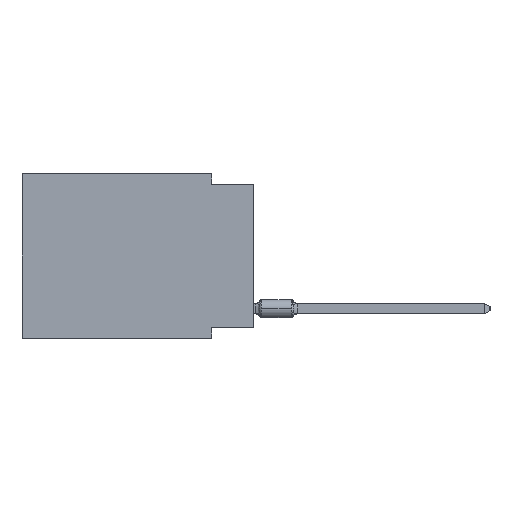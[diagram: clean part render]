
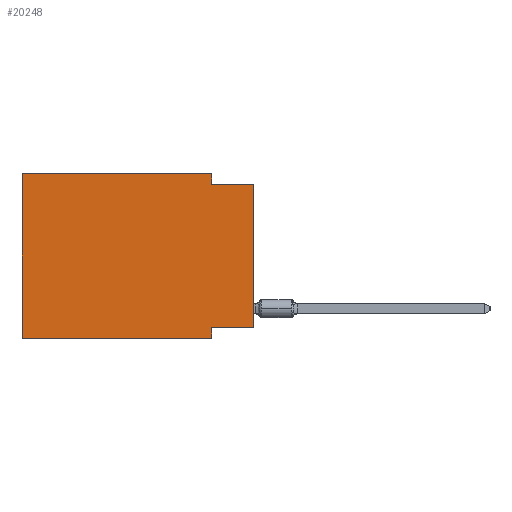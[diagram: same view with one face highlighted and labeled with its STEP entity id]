
A CAD part, left-side view. The second image highlights one B-rep face of the part: STEP entity #20248.
In plain terms, the highlighted planar face has unit normal (-1, 0, 0).
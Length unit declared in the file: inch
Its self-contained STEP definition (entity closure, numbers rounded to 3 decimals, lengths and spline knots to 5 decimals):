
#66 = LINE ( 'NONE', #49662, #8946 ) ;
#1656 = LINE ( 'NONE', #46971, #32949 ) ;
#2371 = DIRECTION ( 'NONE',  ( 0., 0., -1. ) ) ;
#3465 = DIRECTION ( 'NONE',  ( 0., 1., 0. ) ) ;
#4087 = ORIENTED_EDGE ( 'NONE', *, *, #4797, .F. ) ;
#4797 = EDGE_CURVE ( 'NONE', #6938, #42420, #9261, .T. ) ;
#4893 = FACE_OUTER_BOUND ( 'NONE', #39139, .T. ) ;
#5506 = DIRECTION ( 'NONE',  ( 0., -1., 0. ) ) ;
#6291 = ORIENTED_EDGE ( 'NONE', *, *, #38632, .F. ) ;
#6938 = VERTEX_POINT ( 'NONE', #12622 ) ;
#8655 = AXIS2_PLACEMENT_3D ( 'NONE', #35612, #22240, #2371 ) ;
#8905 = ORIENTED_EDGE ( 'NONE', *, *, #30160, .T. ) ;
#8946 = VECTOR ( 'NONE', #22973, 39.37008 ) ;
#9261 = LINE ( 'NONE', #36220, #21050 ) ;
#9319 = DIRECTION ( 'NONE',  ( 0., 0., 1. ) ) ;
#9349 = EDGE_CURVE ( 'NONE', #19573, #6938, #29461, .T. ) ;
#10057 = LINE ( 'NONE', #36007, #34071 ) ;
#11770 = VECTOR ( 'NONE', #9319, 39.37008 ) ;
#12622 = CARTESIAN_POINT ( 'NONE',  ( 0., 0.55, 0. ) ) ;
#14518 = VECTOR ( 'NONE', #37254, 39.37008 ) ;
#14644 = CARTESIAN_POINT ( 'NONE',  ( 0., 0., -0.365 ) ) ;
#15136 = CARTESIAN_POINT ( 'NONE',  ( 0., 0.1, -0.39 ) ) ;
#18146 = DIRECTION ( 'NONE',  ( 0., 0., -1. ) ) ;
#19573 = VERTEX_POINT ( 'NONE', #45070 ) ;
#20248 = ADVANCED_FACE ( 'NONE', ( #4893 ), #46694, .F. ) ;
#20419 = VECTOR ( 'NONE', #18146, 39.37008 ) ;
#21050 = VECTOR ( 'NONE', #5506, 39.37008 ) ;
#22240 = DIRECTION ( 'NONE',  ( 1., 0., 0. ) ) ;
#22973 = DIRECTION ( 'NONE',  ( 0., -1., 0. ) ) ;
#24551 = ORIENTED_EDGE ( 'NONE', *, *, #9349, .F. ) ;
#24905 = VERTEX_POINT ( 'NONE', #47144 ) ;
#27071 = VERTEX_POINT ( 'NONE', #14644 ) ;
#28053 = VECTOR ( 'NONE', #3465, 39.37008 ) ;
#28501 = VERTEX_POINT ( 'NONE', #47668 ) ;
#28958 = LINE ( 'NONE', #48346, #14518 ) ;
#29109 = EDGE_CURVE ( 'NONE', #27071, #47621, #37956, .T. ) ;
#29461 = LINE ( 'NONE', #37009, #11770 ) ;
#30139 = CARTESIAN_POINT ( 'NONE',  ( 0., 0., -0.365 ) ) ;
#30160 = EDGE_CURVE ( 'NONE', #27071, #24905, #1656, .T. ) ;
#31228 = EDGE_CURVE ( 'NONE', #42420, #28501, #28958, .T. ) ;
#32145 = VERTEX_POINT ( 'NONE', #15136 ) ;
#32216 = DIRECTION ( 'NONE',  ( 0., -1., 0. ) ) ;
#32949 = VECTOR ( 'NONE', #38247, 39.37008 ) ;
#33582 = EDGE_CURVE ( 'NONE', #28501, #24905, #66, .T. ) ;
#34071 = VECTOR ( 'NONE', #32216, 39.37008 ) ;
#35612 = CARTESIAN_POINT ( 'NONE',  ( 0., 0.55, 0. ) ) ;
#35768 = ORIENTED_EDGE ( 'NONE', *, *, #31228, .F. ) ;
#35792 = ORIENTED_EDGE ( 'NONE', *, *, #29109, .F. ) ;
#36007 = CARTESIAN_POINT ( 'NONE',  ( 0., 0.55, -0.39 ) ) ;
#36220 = CARTESIAN_POINT ( 'NONE',  ( 0., 0.55, 0. ) ) ;
#37009 = CARTESIAN_POINT ( 'NONE',  ( 0., 0.55, 0. ) ) ;
#37060 = ORIENTED_EDGE ( 'NONE', *, *, #46050, .T. ) ;
#37254 = DIRECTION ( 'NONE',  ( 0., 0., -1. ) ) ;
#37956 = LINE ( 'NONE', #30139, #28053 ) ;
#38247 = DIRECTION ( 'NONE',  ( 0., 0., 1. ) ) ;
#38632 = EDGE_CURVE ( 'NONE', #47621, #32145, #48642, .T. ) ;
#39139 = EDGE_LOOP ( 'NONE', ( #8905, #40990, #35768, #4087, #24551, #37060, #6291, #35792 ) ) ;
#40990 = ORIENTED_EDGE ( 'NONE', *, *, #33582, .F. ) ;
#41322 = CARTESIAN_POINT ( 'NONE',  ( 0., 0.1, -0.39 ) ) ;
#42420 = VERTEX_POINT ( 'NONE', #47113 ) ;
#45070 = CARTESIAN_POINT ( 'NONE',  ( 0., 0.55, -0.39 ) ) ;
#46050 = EDGE_CURVE ( 'NONE', #19573, #32145, #10057, .T. ) ;
#46694 = PLANE ( 'NONE',  #8655 ) ;
#46971 = CARTESIAN_POINT ( 'NONE',  ( 0., 0., 0. ) ) ;
#47113 = CARTESIAN_POINT ( 'NONE',  ( 0., 0.1, 0. ) ) ;
#47144 = CARTESIAN_POINT ( 'NONE',  ( 0., 0., -0.025 ) ) ;
#47621 = VERTEX_POINT ( 'NONE', #48517 ) ;
#47668 = CARTESIAN_POINT ( 'NONE',  ( 0., 0.1, -0.025 ) ) ;
#48346 = CARTESIAN_POINT ( 'NONE',  ( 0., 0.1, 0. ) ) ;
#48517 = CARTESIAN_POINT ( 'NONE',  ( 0., 0.1, -0.365 ) ) ;
#48642 = LINE ( 'NONE', #41322, #20419 ) ;
#49662 = CARTESIAN_POINT ( 'NONE',  ( 0., 0., -0.025 ) ) ;
